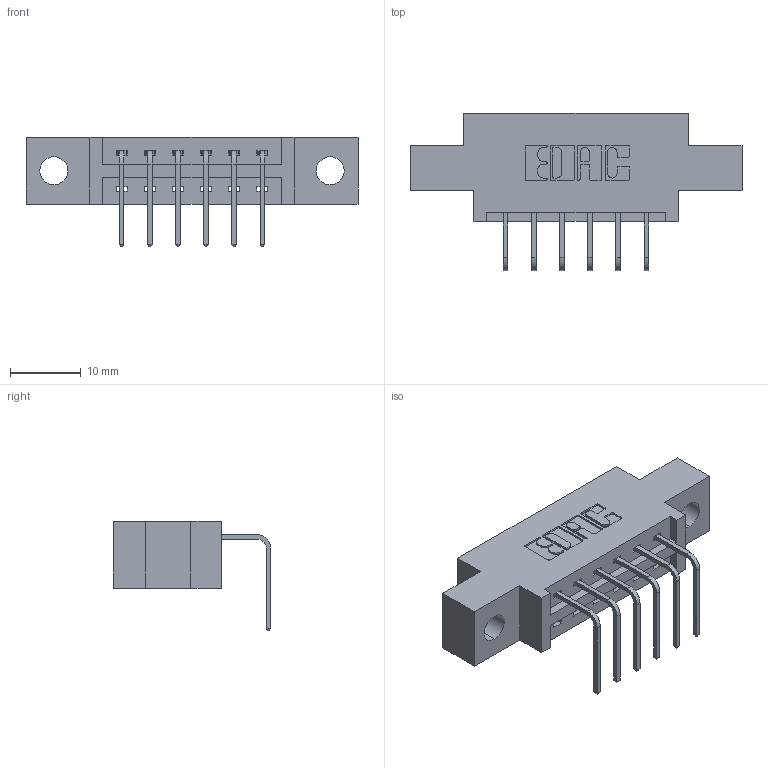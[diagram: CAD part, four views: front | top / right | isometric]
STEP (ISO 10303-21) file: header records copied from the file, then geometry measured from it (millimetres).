
FILE_DESCRIPTION (( 'STEP AP203' ), '1' );
FILE_NAME ('387-006-558-604.STEP', '2019-10-07T15:42:53', ( '' ), ( '' ), 'SwSTEP 2.0', 'SolidWorks 2016', '' );
FILE_SCHEMA (( 'CONFIG_CONTROL_DESIGN' ));
Length unit declared in the file: inch
Products named in the file (3): 345-292-001_558 Tail - 2; 387-006-558-604; 337 Part_0.170 Offset - 0.156 Dia-TH
Assembly tree (7 placements, depth 2):
  387-006-558-604
    337 Part_0.170 Offset - 0.156 Dia-TH
    345-292-001_558 Tail - 2  x6
Bounding box: 46.79 x 22.17 x 15.37 mm (x, y, z)
Volume: 4226.8 mm3; surface area: 4182.5 mm2
Topology: 7 solids, 7 shells, 502 faces, 1487 edges, 982 vertices
Faces by surface type: plane 362, cylinder 140
Entity records: 9335 total; most frequent: CARTESIAN_POINT 1632, ORIENTED_EDGE 1574, DIRECTION 1447, EDGE_CURVE 787, LINE 659, VECTOR 659, VERTEX_POINT 522, AXIS2_PLACEMENT_3D 394
